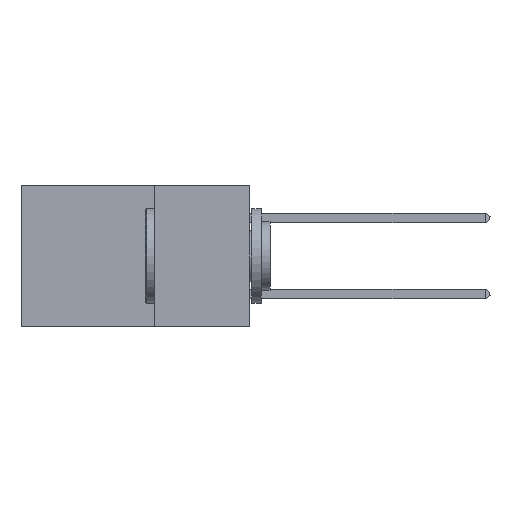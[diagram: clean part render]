
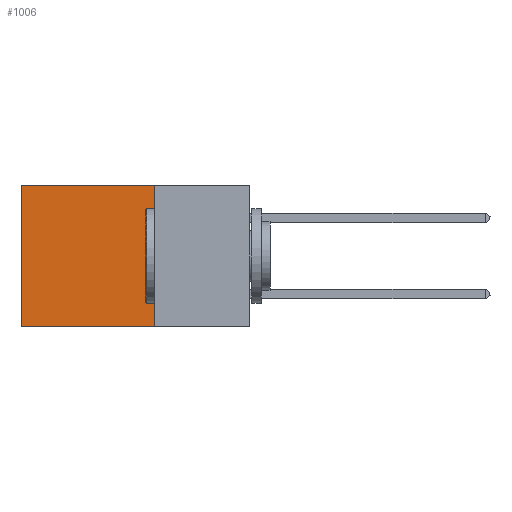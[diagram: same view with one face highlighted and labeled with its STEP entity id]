
A CAD part, left-side view. The second image highlights one B-rep face of the part: STEP entity #1006.
In plain terms, the highlighted planar face has unit normal (-1, 0, 0).
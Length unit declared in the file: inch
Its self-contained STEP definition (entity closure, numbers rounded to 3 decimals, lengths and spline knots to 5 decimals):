
#167 = LINE ( 'NONE', #21717, #21631 ) ;
#1006 = ADVANCED_FACE ( 'NONE', ( #12208 ), #25172, .F. ) ;
#1267 = CARTESIAN_POINT ( 'NONE',  ( 0.2875, 0.6, -0.37 ) ) ;
#1396 = VERTEX_POINT ( 'NONE', #5938 ) ;
#1891 = CARTESIAN_POINT ( 'NONE',  ( 0.2875, 0.25, -0.37 ) ) ;
#2195 = ORIENTED_EDGE ( 'NONE', *, *, #18247, .T. ) ;
#2766 = DIRECTION ( 'NONE',  ( 0., 0., -1. ) ) ;
#3692 = ORIENTED_EDGE ( 'NONE', *, *, #14780, .F. ) ;
#4934 = DIRECTION ( 'NONE',  ( 0., 1., 0. ) ) ;
#5938 = CARTESIAN_POINT ( 'NONE',  ( 0.2875, 0.6, 0. ) ) ;
#6973 = VECTOR ( 'NONE', #27344, 39.37008 ) ;
#7992 = LINE ( 'NONE', #28264, #23750 ) ;
#8138 = CARTESIAN_POINT ( 'NONE',  ( 0.2875, 0.25, -0.37 ) ) ;
#8436 = CARTESIAN_POINT ( 'NONE',  ( 0.2875, 0.25, 0. ) ) ;
#10038 = EDGE_CURVE ( 'NONE', #31846, #25479, #19236, .T. ) ;
#12208 = FACE_OUTER_BOUND ( 'NONE', #13594, .T. ) ;
#12981 = ORIENTED_EDGE ( 'NONE', *, *, #17206, .T. ) ;
#13594 = EDGE_LOOP ( 'NONE', ( #2195, #22953, #3692, #12981 ) ) ;
#14156 = CARTESIAN_POINT ( 'NONE',  ( 0.2875, 0.25, 0. ) ) ;
#14780 = EDGE_CURVE ( 'NONE', #27245, #31846, #27457, .T. ) ;
#17206 = EDGE_CURVE ( 'NONE', #27245, #1396, #167, .T. ) ;
#18247 = EDGE_CURVE ( 'NONE', #1396, #25479, #7992, .T. ) ;
#19236 = LINE ( 'NONE', #8138, #6973 ) ;
#21631 = VECTOR ( 'NONE', #4934, 39.37008 ) ;
#21717 = CARTESIAN_POINT ( 'NONE',  ( 0.2875, 0.25, 0. ) ) ;
#22953 = ORIENTED_EDGE ( 'NONE', *, *, #10038, .F. ) ;
#23048 = AXIS2_PLACEMENT_3D ( 'NONE', #8436, #27998, #36082 ) ;
#23750 = VECTOR ( 'NONE', #2766, 39.37008 ) ;
#25172 = PLANE ( 'NONE',  #23048 ) ;
#25479 = VERTEX_POINT ( 'NONE', #1267 ) ;
#26580 = VECTOR ( 'NONE', #27290, 39.37008 ) ;
#27245 = VERTEX_POINT ( 'NONE', #14156 ) ;
#27290 = DIRECTION ( 'NONE',  ( 0., 0., -1. ) ) ;
#27344 = DIRECTION ( 'NONE',  ( 0., 1., 0. ) ) ;
#27457 = LINE ( 'NONE', #35583, #26580 ) ;
#27998 = DIRECTION ( 'NONE',  ( 1., 0., 0. ) ) ;
#28264 = CARTESIAN_POINT ( 'NONE',  ( 0.2875, 0.6, 0. ) ) ;
#31846 = VERTEX_POINT ( 'NONE', #1891 ) ;
#35583 = CARTESIAN_POINT ( 'NONE',  ( 0.2875, 0.25, 0. ) ) ;
#36082 = DIRECTION ( 'NONE',  ( 0., 0., -1. ) ) ;
